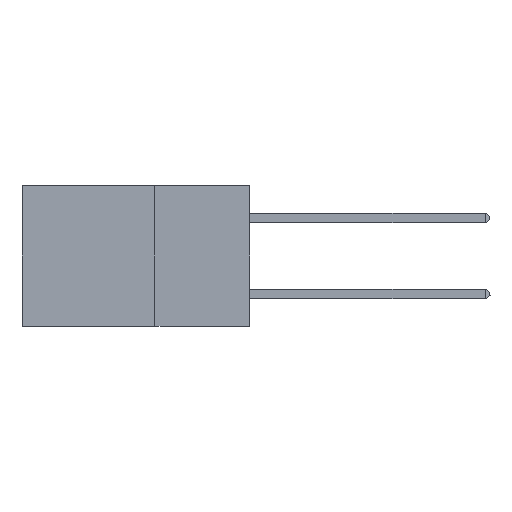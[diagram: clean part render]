
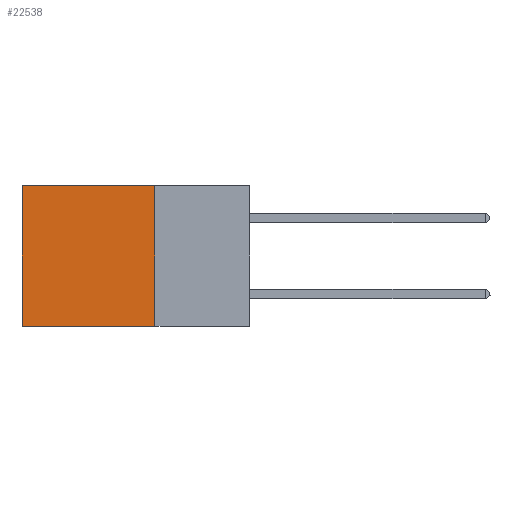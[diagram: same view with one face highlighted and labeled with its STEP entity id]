
A CAD part, left-side view. The second image highlights one B-rep face of the part: STEP entity #22538.
In plain terms, the highlighted planar face has unit normal (-1, 0, 0).
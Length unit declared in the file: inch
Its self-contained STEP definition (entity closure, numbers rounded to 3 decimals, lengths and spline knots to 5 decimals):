
#1351 = EDGE_LOOP ( 'NONE', ( #23245, #15310, #16095, #25987 ) ) ;
#1919 = CARTESIAN_POINT ( 'NONE',  ( 0.2875, 0.25, -0.37 ) ) ;
#3157 = CARTESIAN_POINT ( 'NONE',  ( 0.2875, 0.25, 0. ) ) ;
#4498 = EDGE_CURVE ( 'NONE', #15956, #10109, #30731, .T. ) ;
#5422 = CARTESIAN_POINT ( 'NONE',  ( 0.2875, 0.6, -0.37 ) ) ;
#5548 = LINE ( 'NONE', #25900, #27841 ) ;
#5736 = EDGE_CURVE ( 'NONE', #18924, #15956, #12802, .T. ) ;
#8094 = CARTESIAN_POINT ( 'NONE',  ( 0.2875, 0.6, 0. ) ) ;
#8911 = CARTESIAN_POINT ( 'NONE',  ( 0.2875, 0.25, -0.37 ) ) ;
#10109 = VERTEX_POINT ( 'NONE', #5422 ) ;
#12802 = LINE ( 'NONE', #25539, #13200 ) ;
#12827 = DIRECTION ( 'NONE',  ( 0., 1., 0. ) ) ;
#13200 = VECTOR ( 'NONE', #28442, 39.37008 ) ;
#13262 = VECTOR ( 'NONE', #31430, 39.37008 ) ;
#14630 = CARTESIAN_POINT ( 'NONE',  ( 0.2875, 0.6, 0. ) ) ;
#15310 = ORIENTED_EDGE ( 'NONE', *, *, #4498, .F. ) ;
#15667 = AXIS2_PLACEMENT_3D ( 'NONE', #18839, #24095, #18613 ) ;
#15956 = VERTEX_POINT ( 'NONE', #8911 ) ;
#16095 = ORIENTED_EDGE ( 'NONE', *, *, #5736, .F. ) ;
#16164 = VECTOR ( 'NONE', #17710, 39.37008 ) ;
#17005 = EDGE_CURVE ( 'NONE', #17252, #10109, #27869, .T. ) ;
#17252 = VERTEX_POINT ( 'NONE', #14630 ) ;
#17710 = DIRECTION ( 'NONE',  ( 0., 1., 0. ) ) ;
#18613 = DIRECTION ( 'NONE',  ( 0., 0., -1. ) ) ;
#18839 = CARTESIAN_POINT ( 'NONE',  ( 0.2875, 0.25, 0. ) ) ;
#18924 = VERTEX_POINT ( 'NONE', #3157 ) ;
#22538 = ADVANCED_FACE ( 'NONE', ( #23955 ), #26770, .F. ) ;
#23245 = ORIENTED_EDGE ( 'NONE', *, *, #17005, .T. ) ;
#23955 = FACE_OUTER_BOUND ( 'NONE', #1351, .T. ) ;
#24095 = DIRECTION ( 'NONE',  ( 1., 0., 0. ) ) ;
#25539 = CARTESIAN_POINT ( 'NONE',  ( 0.2875, 0.25, 0. ) ) ;
#25900 = CARTESIAN_POINT ( 'NONE',  ( 0.2875, 0.25, 0. ) ) ;
#25987 = ORIENTED_EDGE ( 'NONE', *, *, #26063, .T. ) ;
#26063 = EDGE_CURVE ( 'NONE', #18924, #17252, #5548, .T. ) ;
#26770 = PLANE ( 'NONE',  #15667 ) ;
#27841 = VECTOR ( 'NONE', #12827, 39.37008 ) ;
#27869 = LINE ( 'NONE', #8094, #13262 ) ;
#28442 = DIRECTION ( 'NONE',  ( 0., 0., -1. ) ) ;
#30731 = LINE ( 'NONE', #1919, #16164 ) ;
#31430 = DIRECTION ( 'NONE',  ( 0., 0., -1. ) ) ;
